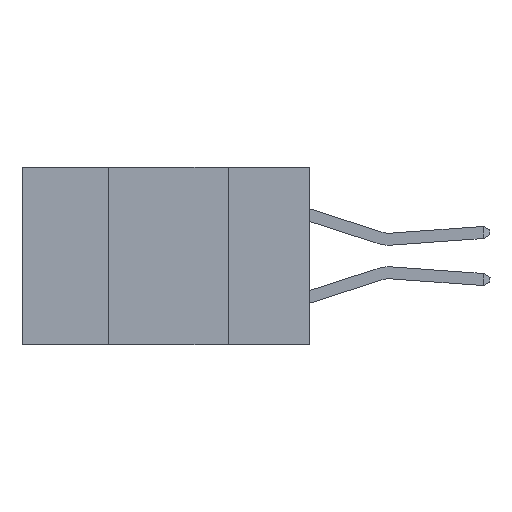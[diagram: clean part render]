
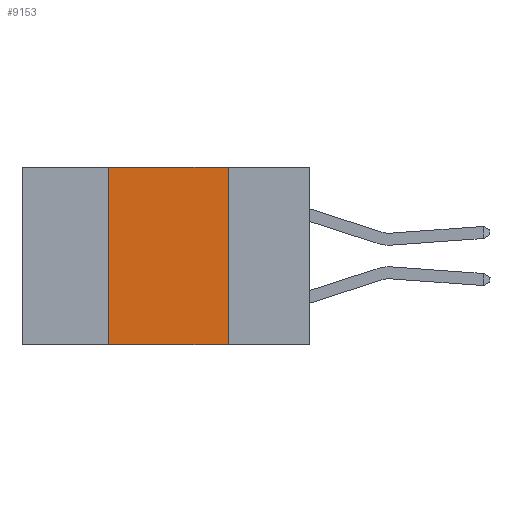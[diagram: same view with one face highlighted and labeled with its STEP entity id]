
A CAD part, left-side view. The second image highlights one B-rep face of the part: STEP entity #9153.
In plain terms, the highlighted planar face has unit normal (-1, 0, 0).
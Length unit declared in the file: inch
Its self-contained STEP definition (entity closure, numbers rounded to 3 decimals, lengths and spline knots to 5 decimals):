
#95 = CARTESIAN_POINT ( 'NONE',  ( 0., 0.17, 0. ) ) ;
#391 = VERTEX_POINT ( 'NONE', #5957 ) ;
#1069 = VECTOR ( 'NONE', #2086, 39.37008 ) ;
#1114 = LINE ( 'NONE', #6279, #3767 ) ;
#1357 = CARTESIAN_POINT ( 'NONE',  ( 0., 0.42, -0.37 ) ) ;
#2086 = DIRECTION ( 'NONE',  ( 0., -1., 0. ) ) ;
#2187 = LINE ( 'NONE', #2970, #1069 ) ;
#2275 = ORIENTED_EDGE ( 'NONE', *, *, #4132, .F. ) ;
#2771 = DIRECTION ( 'NONE',  ( 0., 0., -1. ) ) ;
#2970 = CARTESIAN_POINT ( 'NONE',  ( 0., 0.6, 0. ) ) ;
#3325 = VECTOR ( 'NONE', #9358, 39.37008 ) ;
#3496 = ORIENTED_EDGE ( 'NONE', *, *, #4079, .F. ) ;
#3767 = VECTOR ( 'NONE', #5527, 39.37008 ) ;
#4079 = EDGE_CURVE ( 'NONE', #6699, #5632, #7558, .T. ) ;
#4132 = EDGE_CURVE ( 'NONE', #5047, #391, #7290, .T. ) ;
#4403 = ORIENTED_EDGE ( 'NONE', *, *, #6823, .F. ) ;
#4613 = DIRECTION ( 'NONE',  ( 0., 0., -1. ) ) ;
#4642 = CARTESIAN_POINT ( 'NONE',  ( 0., 0.17, -0.37 ) ) ;
#5047 = VERTEX_POINT ( 'NONE', #95 ) ;
#5061 = CARTESIAN_POINT ( 'NONE',  ( 0., 0.6, 0. ) ) ;
#5102 = PLANE ( 'NONE',  #6979 ) ;
#5527 = DIRECTION ( 'NONE',  ( 0., -1., 0. ) ) ;
#5632 = VERTEX_POINT ( 'NONE', #7386 ) ;
#5957 = CARTESIAN_POINT ( 'NONE',  ( 0., 0.17, -0.37 ) ) ;
#6176 = ORIENTED_EDGE ( 'NONE', *, *, #10293, .T. ) ;
#6279 = CARTESIAN_POINT ( 'NONE',  ( 0., 0.6, -0.37 ) ) ;
#6699 = VERTEX_POINT ( 'NONE', #7462 ) ;
#6789 = VECTOR ( 'NONE', #4613, 39.37008 ) ;
#6823 = EDGE_CURVE ( 'NONE', #5632, #5047, #2187, .T. ) ;
#6979 = AXIS2_PLACEMENT_3D ( 'NONE', #5061, #7542, #2771 ) ;
#7290 = LINE ( 'NONE', #4642, #6789 ) ;
#7386 = CARTESIAN_POINT ( 'NONE',  ( 0., 0.42, 0. ) ) ;
#7462 = CARTESIAN_POINT ( 'NONE',  ( 0., 0.42, -0.37 ) ) ;
#7542 = DIRECTION ( 'NONE',  ( 1., 0., 0. ) ) ;
#7558 = LINE ( 'NONE', #1357, #3325 ) ;
#9153 = ADVANCED_FACE ( 'NONE', ( #9353 ), #5102, .F. ) ;
#9353 = FACE_OUTER_BOUND ( 'NONE', #10066, .T. ) ;
#9358 = DIRECTION ( 'NONE',  ( 0., 0., 1. ) ) ;
#10066 = EDGE_LOOP ( 'NONE', ( #2275, #4403, #3496, #6176 ) ) ;
#10293 = EDGE_CURVE ( 'NONE', #6699, #391, #1114, .T. ) ;
